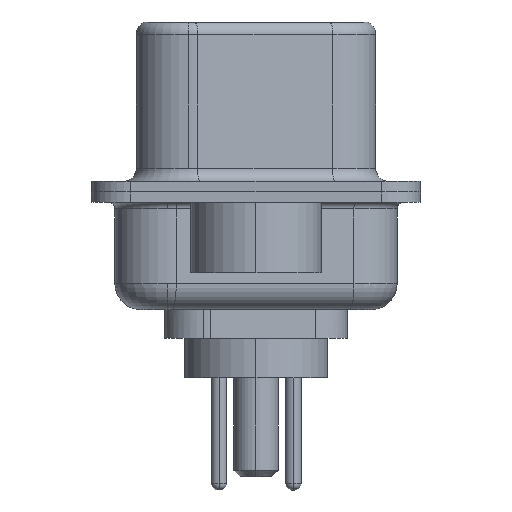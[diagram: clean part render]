
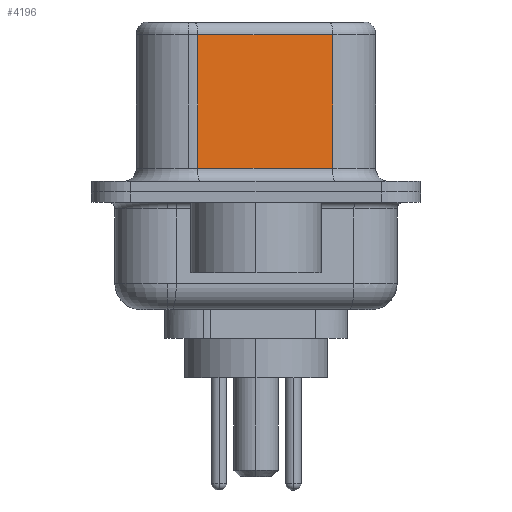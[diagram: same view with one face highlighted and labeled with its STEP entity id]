
A CAD part, left-side view. The second image highlights one B-rep face of the part: STEP entity #4196.
In plain terms, the highlighted planar face has unit normal (-0.985, -0.174, 0).
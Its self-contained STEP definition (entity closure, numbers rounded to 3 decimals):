
#70 = FACE_OUTER_BOUND ( 'NONE', #4943, .T. ) ;
#292 = ORIENTED_EDGE ( 'NONE', *, *, #17785, .T. ) ;
#1264 = CARTESIAN_POINT ( 'NONE',  ( 4.585, -2.927, 6.52 ) ) ;
#2698 = VERTEX_POINT ( 'NONE', #19399 ) ;
#2707 = VECTOR ( 'NONE', #3322, 1000. ) ;
#3262 = DIRECTION ( 'NONE',  ( 0.174, -0.985, 0. ) ) ;
#3322 = DIRECTION ( 'NONE',  ( -0.174, 0.985, 0. ) ) ;
#4196 = ADVANCED_FACE ( 'NONE', ( #70 ), #7653, .F. ) ;
#4906 = ORIENTED_EDGE ( 'NONE', *, *, #20140, .T. ) ;
#4943 = EDGE_LOOP ( 'NONE', ( #17961, #4906, #292, #5681 ) ) ;
#5681 = ORIENTED_EDGE ( 'NONE', *, *, #15267, .T. ) ;
#6014 = DIRECTION ( 'NONE',  ( 0., 0., -1. ) ) ;
#6718 = LINE ( 'NONE', #17000, #2707 ) ;
#7559 = LINE ( 'NONE', #8501, #15015 ) ;
#7653 = PLANE ( 'NONE',  #11349 ) ;
#8055 = CARTESIAN_POINT ( 'NONE',  ( 4.585, -2.927, 0.9 ) ) ;
#8501 = CARTESIAN_POINT ( 'NONE',  ( 4.585, -2.927, 0.9 ) ) ;
#8848 = VECTOR ( 'NONE', #15477, 1000. ) ;
#10486 = VERTEX_POINT ( 'NONE', #8055 ) ;
#11349 = AXIS2_PLACEMENT_3D ( 'NONE', #1264, #11974, #14344 ) ;
#11974 = DIRECTION ( 'NONE',  ( 0.985, 0.174, 0. ) ) ;
#12048 = VECTOR ( 'NONE', #6014, 1000. ) ;
#12062 = CARTESIAN_POINT ( 'NONE',  ( 4.585, -2.927, 6.52 ) ) ;
#13647 = LINE ( 'NONE', #14536, #12048 ) ;
#13855 = LINE ( 'NONE', #12062, #8848 ) ;
#14344 = DIRECTION ( 'NONE',  ( -0.174, 0.985, 0. ) ) ;
#14536 = CARTESIAN_POINT ( 'NONE',  ( 3.675, 2.233, 6.52 ) ) ;
#14812 = VERTEX_POINT ( 'NONE', #16696 ) ;
#15015 = VECTOR ( 'NONE', #3262, 1000. ) ;
#15267 = EDGE_CURVE ( 'NONE', #2698, #10486, #7559, .T. ) ;
#15477 = DIRECTION ( 'NONE',  ( 0., 0., -1. ) ) ;
#16170 = CARTESIAN_POINT ( 'NONE',  ( 4.585, -2.927, 6.02 ) ) ;
#16355 = VERTEX_POINT ( 'NONE', #16170 ) ;
#16696 = CARTESIAN_POINT ( 'NONE',  ( 3.675, 2.233, 6.02 ) ) ;
#17000 = CARTESIAN_POINT ( 'NONE',  ( 4.585, -2.927, 6.02 ) ) ;
#17785 = EDGE_CURVE ( 'NONE', #14812, #2698, #13647, .T. ) ;
#17961 = ORIENTED_EDGE ( 'NONE', *, *, #19054, .F. ) ;
#19054 = EDGE_CURVE ( 'NONE', #16355, #10486, #13855, .T. ) ;
#19399 = CARTESIAN_POINT ( 'NONE',  ( 3.675, 2.233, 0.9 ) ) ;
#20140 = EDGE_CURVE ( 'NONE', #16355, #14812, #6718, .T. ) ;
